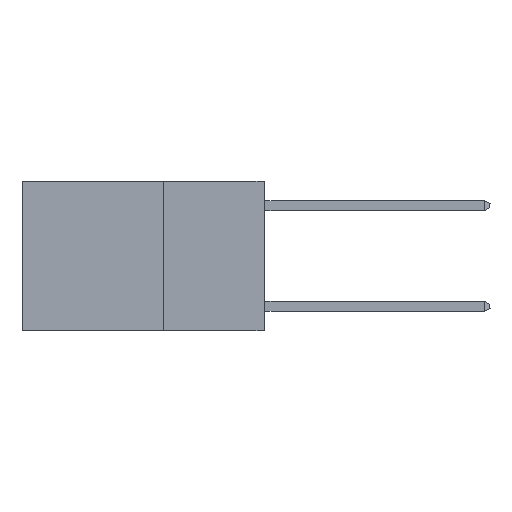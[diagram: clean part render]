
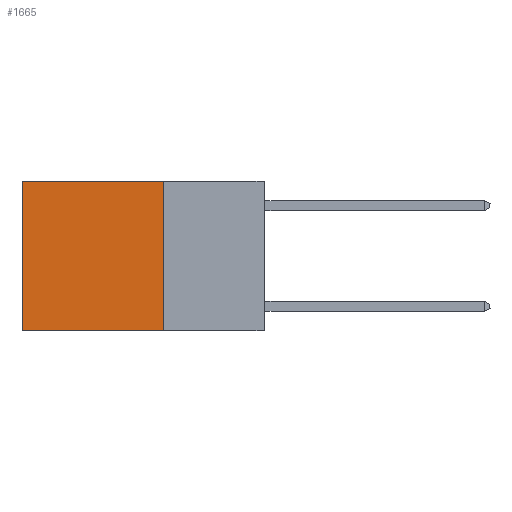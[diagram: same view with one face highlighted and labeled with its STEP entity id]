
A CAD part, left-side view. The second image highlights one B-rep face of the part: STEP entity #1665.
In plain terms, the highlighted planar face has unit normal (-1, 0, 0).
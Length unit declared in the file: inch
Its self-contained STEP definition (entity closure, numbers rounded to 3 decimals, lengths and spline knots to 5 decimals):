
#160 = CARTESIAN_POINT ( 'NONE',  ( 0.2625, 0.25, -0.37 ) ) ;
#1291 = EDGE_LOOP ( 'NONE', ( #10219, #7285, #3897, #2622 ) ) ;
#1500 = VECTOR ( 'NONE', #5708, 39.37008 ) ;
#1630 = LINE ( 'NONE', #10967, #3838 ) ;
#1665 = ADVANCED_FACE ( 'NONE', ( #7852 ), #5076, .F. ) ;
#1683 = CARTESIAN_POINT ( 'NONE',  ( 0.2625, 0.25, 0. ) ) ;
#2359 = CARTESIAN_POINT ( 'NONE',  ( 0.2625, 0.6, 0. ) ) ;
#2622 = ORIENTED_EDGE ( 'NONE', *, *, #7415, .T. ) ;
#2711 = VECTOR ( 'NONE', #4415, 39.37008 ) ;
#3838 = VECTOR ( 'NONE', #10724, 39.37008 ) ;
#3897 = ORIENTED_EDGE ( 'NONE', *, *, #6082, .F. ) ;
#4187 = DIRECTION ( 'NONE',  ( 0., 0., -1. ) ) ;
#4317 = CARTESIAN_POINT ( 'NONE',  ( 0.2625, 0.25, 0. ) ) ;
#4415 = DIRECTION ( 'NONE',  ( 0., 0., -1. ) ) ;
#5076 = PLANE ( 'NONE',  #6879 ) ;
#5438 = LINE ( 'NONE', #6334, #2711 ) ;
#5630 = LINE ( 'NONE', #160, #10876 ) ;
#5708 = DIRECTION ( 'NONE',  ( 0., 1., 0. ) ) ;
#5750 = VERTEX_POINT ( 'NONE', #6121 ) ;
#5775 = CARTESIAN_POINT ( 'NONE',  ( 0.2625, 0.25, 0. ) ) ;
#5847 = LINE ( 'NONE', #5775, #1500 ) ;
#6082 = EDGE_CURVE ( 'NONE', #8446, #10569, #1630, .T. ) ;
#6121 = CARTESIAN_POINT ( 'NONE',  ( 0.2625, 0.6, -0.37 ) ) ;
#6334 = CARTESIAN_POINT ( 'NONE',  ( 0.2625, 0.6, 0. ) ) ;
#6341 = DIRECTION ( 'NONE',  ( 0., 1., 0. ) ) ;
#6879 = AXIS2_PLACEMENT_3D ( 'NONE', #4317, #7017, #4187 ) ;
#6908 = EDGE_CURVE ( 'NONE', #11727, #5750, #5438, .T. ) ;
#7017 = DIRECTION ( 'NONE',  ( 1., 0., 0. ) ) ;
#7285 = ORIENTED_EDGE ( 'NONE', *, *, #8593, .F. ) ;
#7415 = EDGE_CURVE ( 'NONE', #8446, #11727, #5847, .T. ) ;
#7852 = FACE_OUTER_BOUND ( 'NONE', #1291, .T. ) ;
#8446 = VERTEX_POINT ( 'NONE', #1683 ) ;
#8593 = EDGE_CURVE ( 'NONE', #10569, #5750, #5630, .T. ) ;
#8624 = CARTESIAN_POINT ( 'NONE',  ( 0.2625, 0.25, -0.37 ) ) ;
#10219 = ORIENTED_EDGE ( 'NONE', *, *, #6908, .T. ) ;
#10569 = VERTEX_POINT ( 'NONE', #8624 ) ;
#10724 = DIRECTION ( 'NONE',  ( 0., 0., -1. ) ) ;
#10876 = VECTOR ( 'NONE', #6341, 39.37008 ) ;
#10967 = CARTESIAN_POINT ( 'NONE',  ( 0.2625, 0.25, 0. ) ) ;
#11727 = VERTEX_POINT ( 'NONE', #2359 ) ;
